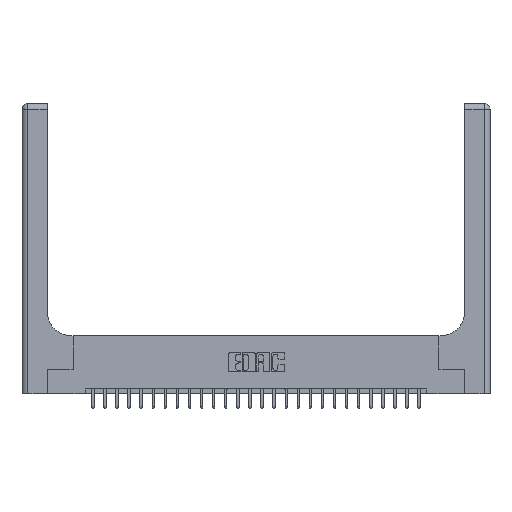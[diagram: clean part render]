
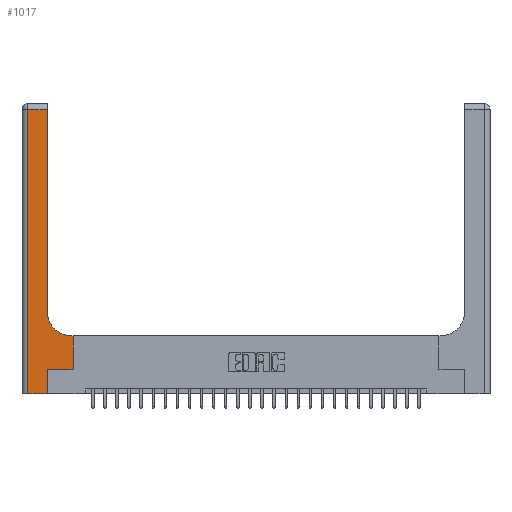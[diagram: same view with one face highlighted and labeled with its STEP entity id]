
A CAD part, top view. The second image highlights one B-rep face of the part: STEP entity #1017.
In plain terms, the highlighted planar face has unit normal (0, 0, 1).
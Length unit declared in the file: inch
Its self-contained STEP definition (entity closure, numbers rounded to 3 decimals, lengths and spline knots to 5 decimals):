
#452 = VECTOR ( 'NONE', #19954, 39.37008 ) ;
#910 = CARTESIAN_POINT ( 'NONE',  ( 0.06, 0., 0.37 ) ) ;
#1017 = ADVANCED_FACE ( 'NONE', ( #20492 ), #14391, .F. ) ;
#1456 = VERTEX_POINT ( 'NONE', #18261 ) ;
#1525 = CARTESIAN_POINT ( 'NONE',  ( 0.265, 0., 0.37 ) ) ;
#1600 = VERTEX_POINT ( 'NONE', #5840 ) ;
#1957 = DIRECTION ( 'NONE',  ( 1., 0., 0. ) ) ;
#2397 = EDGE_CURVE ( 'NONE', #1456, #7990, #21928, .T. ) ;
#2718 = EDGE_CURVE ( 'NONE', #12883, #24579, #10833, .T. ) ;
#3093 = CARTESIAN_POINT ( 'NONE',  ( 0.265, 0., 0.37 ) ) ;
#4314 = DIRECTION ( 'NONE',  ( -1., 0., 0. ) ) ;
#4921 = ORIENTED_EDGE ( 'NONE', *, *, #12903, .T. ) ;
#5724 = CARTESIAN_POINT ( 'NONE',  ( 0.26, 3., 0.37 ) ) ;
#5840 = CARTESIAN_POINT ( 'NONE',  ( 0.26, 2.94, 0.37 ) ) ;
#5931 = VECTOR ( 'NONE', #7589, 39.37008 ) ;
#6001 = EDGE_CURVE ( 'NONE', #7990, #10783, #10200, .T. ) ;
#6067 = ORIENTED_EDGE ( 'NONE', *, *, #14832, .T. ) ;
#6417 = CARTESIAN_POINT ( 'NONE',  ( 0.528, 0.25, 0.37 ) ) ;
#6525 = VECTOR ( 'NONE', #14441, 39.37008 ) ;
#6769 = DIRECTION ( 'NONE',  ( 0., 1., 0. ) ) ;
#7220 = ORIENTED_EDGE ( 'NONE', *, *, #15326, .T. ) ;
#7589 = DIRECTION ( 'NONE',  ( 0., -1., 0. ) ) ;
#7606 = EDGE_CURVE ( 'NONE', #20498, #19605, #25481, .T. ) ;
#7990 = VERTEX_POINT ( 'NONE', #15264 ) ;
#8500 = CARTESIAN_POINT ( 'NONE',  ( 0., 3., 0.37 ) ) ;
#9431 = CARTESIAN_POINT ( 'NONE',  ( 0.528, 0.6, 0.37 ) ) ;
#9912 = LINE ( 'NONE', #10173, #452 ) ;
#10173 = CARTESIAN_POINT ( 'NONE',  ( 0., 2.94, 0.37 ) ) ;
#10200 = LINE ( 'NONE', #6417, #15893 ) ;
#10783 = VERTEX_POINT ( 'NONE', #9431 ) ;
#10833 = CIRCLE ( 'NONE', #25423, 0.25 ) ;
#10933 = LINE ( 'NONE', #3093, #17905 ) ;
#11399 = ORIENTED_EDGE ( 'NONE', *, *, #7606, .T. ) ;
#12457 = ORIENTED_EDGE ( 'NONE', *, *, #2397, .T. ) ;
#12845 = CARTESIAN_POINT ( 'NONE',  ( 0.26, 0.85, 0.37 ) ) ;
#12883 = VERTEX_POINT ( 'NONE', #15779 ) ;
#12903 = EDGE_CURVE ( 'NONE', #24579, #1600, #13555, .T. ) ;
#12977 = ORIENTED_EDGE ( 'NONE', *, *, #17628, .T. ) ;
#13552 = CARTESIAN_POINT ( 'NONE',  ( 0.51, 0.85, 0.37 ) ) ;
#13555 = LINE ( 'NONE', #5724, #24803 ) ;
#13818 = DIRECTION ( 'NONE',  ( 0., 0., -1. ) ) ;
#14314 = LINE ( 'NONE', #21597, #6525 ) ;
#14391 = PLANE ( 'NONE',  #25799 ) ;
#14441 = DIRECTION ( 'NONE',  ( 1., 0., 0. ) ) ;
#14832 = EDGE_CURVE ( 'NONE', #19605, #17841, #14314, .T. ) ;
#15264 = CARTESIAN_POINT ( 'NONE',  ( 0.528, 0.25, 0.37 ) ) ;
#15326 = EDGE_CURVE ( 'NONE', #10783, #12883, #21448, .T. ) ;
#15779 = CARTESIAN_POINT ( 'NONE',  ( 0.51, 0.6, 0.37 ) ) ;
#15893 = VECTOR ( 'NONE', #22208, 39.37008 ) ;
#16471 = DIRECTION ( 'NONE',  ( 0., 0., -1. ) ) ;
#16504 = CARTESIAN_POINT ( 'NONE',  ( 0.06, 2.94, 0.37 ) ) ;
#17542 = CARTESIAN_POINT ( 'NONE',  ( 0.26, 0.6, 0.37 ) ) ;
#17628 = EDGE_CURVE ( 'NONE', #17841, #1456, #10933, .T. ) ;
#17763 = CARTESIAN_POINT ( 'NONE',  ( 0.265, 0.25, 0.37 ) ) ;
#17841 = VERTEX_POINT ( 'NONE', #1525 ) ;
#17853 = DIRECTION ( 'NONE',  ( 1., 0., 0. ) ) ;
#17905 = VECTOR ( 'NONE', #6769, 39.37008 ) ;
#18151 = ORIENTED_EDGE ( 'NONE', *, *, #2718, .T. ) ;
#18261 = CARTESIAN_POINT ( 'NONE',  ( 0.265, 0.25, 0.37 ) ) ;
#19363 = DIRECTION ( 'NONE',  ( -1., 0., 0. ) ) ;
#19440 = EDGE_LOOP ( 'NONE', ( #4921, #23447, #11399, #6067, #12977, #12457, #25476, #7220, #18151 ) ) ;
#19605 = VERTEX_POINT ( 'NONE', #910 ) ;
#19954 = DIRECTION ( 'NONE',  ( -1., 0., 0. ) ) ;
#20492 = FACE_OUTER_BOUND ( 'NONE', #19440, .T. ) ;
#20498 = VERTEX_POINT ( 'NONE', #16504 ) ;
#21099 = EDGE_CURVE ( 'NONE', #1600, #20498, #9912, .T. ) ;
#21163 = CARTESIAN_POINT ( 'NONE',  ( 0.06, 3., 0.37 ) ) ;
#21448 = LINE ( 'NONE', #17542, #24057 ) ;
#21597 = CARTESIAN_POINT ( 'NONE',  ( 0., 0., 0.37 ) ) ;
#21928 = LINE ( 'NONE', #17763, #24983 ) ;
#22208 = DIRECTION ( 'NONE',  ( 0., 1., 0. ) ) ;
#23447 = ORIENTED_EDGE ( 'NONE', *, *, #21099, .T. ) ;
#23606 = DIRECTION ( 'NONE',  ( 0., 1., 0. ) ) ;
#24057 = VECTOR ( 'NONE', #19363, 39.37008 ) ;
#24579 = VERTEX_POINT ( 'NONE', #12845 ) ;
#24803 = VECTOR ( 'NONE', #23606, 39.37008 ) ;
#24983 = VECTOR ( 'NONE', #1957, 39.37008 ) ;
#25423 = AXIS2_PLACEMENT_3D ( 'NONE', #13552, #13818, #17853 ) ;
#25476 = ORIENTED_EDGE ( 'NONE', *, *, #6001, .T. ) ;
#25481 = LINE ( 'NONE', #21163, #5931 ) ;
#25799 = AXIS2_PLACEMENT_3D ( 'NONE', #8500, #16471, #4314 ) ;
